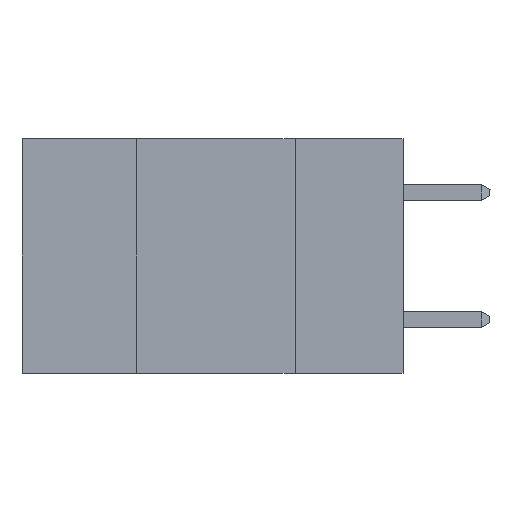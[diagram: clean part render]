
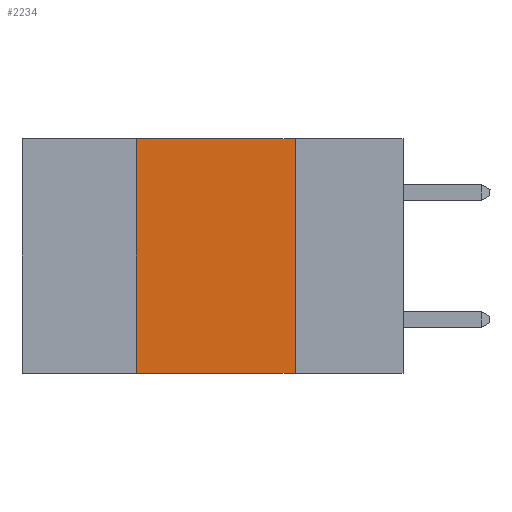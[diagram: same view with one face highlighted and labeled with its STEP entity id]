
A CAD part, left-side view. The second image highlights one B-rep face of the part: STEP entity #2234.
In plain terms, the highlighted planar face has unit normal (-1, 0, 0).
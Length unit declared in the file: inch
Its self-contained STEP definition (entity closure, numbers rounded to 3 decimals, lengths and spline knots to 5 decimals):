
#132 = VERTEX_POINT ( 'NONE', #14257 ) ;
#1269 = VERTEX_POINT ( 'NONE', #9455 ) ;
#1740 = EDGE_CURVE ( 'NONE', #11009, #132, #8018, .T. ) ;
#1852 = LINE ( 'NONE', #11993, #12864 ) ;
#2234 = ADVANCED_FACE ( 'NONE', ( #10199 ), #4156, .F. ) ;
#2387 = AXIS2_PLACEMENT_3D ( 'NONE', #4560, #12291, #14248 ) ;
#2471 = ORIENTED_EDGE ( 'NONE', *, *, #5874, .F. ) ;
#2754 = VECTOR ( 'NONE', #7797, 39.37008 ) ;
#4027 = ORIENTED_EDGE ( 'NONE', *, *, #1740, .T. ) ;
#4156 = PLANE ( 'NONE',  #2387 ) ;
#4560 = CARTESIAN_POINT ( 'NONE',  ( 0., 0.6, 0. ) ) ;
#4632 = CARTESIAN_POINT ( 'NONE',  ( 0., 0.42, -0.37 ) ) ;
#5562 = EDGE_CURVE ( 'NONE', #11009, #1269, #8735, .T. ) ;
#5874 = EDGE_CURVE ( 'NONE', #1269, #6532, #1852, .T. ) ;
#6008 = VECTOR ( 'NONE', #11986, 39.37008 ) ;
#6532 = VERTEX_POINT ( 'NONE', #12410 ) ;
#7688 = VECTOR ( 'NONE', #9557, 39.37008 ) ;
#7724 = CARTESIAN_POINT ( 'NONE',  ( 0., 0.17, 0. ) ) ;
#7797 = DIRECTION ( 'NONE',  ( 0., 0., 1. ) ) ;
#8018 = LINE ( 'NONE', #8957, #7688 ) ;
#8735 = LINE ( 'NONE', #9008, #2754 ) ;
#8943 = LINE ( 'NONE', #7724, #6008 ) ;
#8957 = CARTESIAN_POINT ( 'NONE',  ( 0., 0.6, -0.37 ) ) ;
#9008 = CARTESIAN_POINT ( 'NONE',  ( 0., 0.42, 0. ) ) ;
#9455 = CARTESIAN_POINT ( 'NONE',  ( 0., 0.42, 0. ) ) ;
#9557 = DIRECTION ( 'NONE',  ( 0., -1., 0. ) ) ;
#10199 = FACE_OUTER_BOUND ( 'NONE', #11178, .T. ) ;
#10869 = ORIENTED_EDGE ( 'NONE', *, *, #11445, .F. ) ;
#11009 = VERTEX_POINT ( 'NONE', #4632 ) ;
#11178 = EDGE_LOOP ( 'NONE', ( #10869, #2471, #12124, #4027 ) ) ;
#11203 = DIRECTION ( 'NONE',  ( 0., -1., 0. ) ) ;
#11445 = EDGE_CURVE ( 'NONE', #6532, #132, #8943, .T. ) ;
#11986 = DIRECTION ( 'NONE',  ( 0., 0., -1. ) ) ;
#11993 = CARTESIAN_POINT ( 'NONE',  ( 0., 0.6, 0. ) ) ;
#12124 = ORIENTED_EDGE ( 'NONE', *, *, #5562, .F. ) ;
#12291 = DIRECTION ( 'NONE',  ( 1., 0., 0. ) ) ;
#12410 = CARTESIAN_POINT ( 'NONE',  ( 0., 0.17, 0. ) ) ;
#12864 = VECTOR ( 'NONE', #11203, 39.37008 ) ;
#14248 = DIRECTION ( 'NONE',  ( 0., 0., -1. ) ) ;
#14257 = CARTESIAN_POINT ( 'NONE',  ( 0., 0.17, -0.37 ) ) ;
